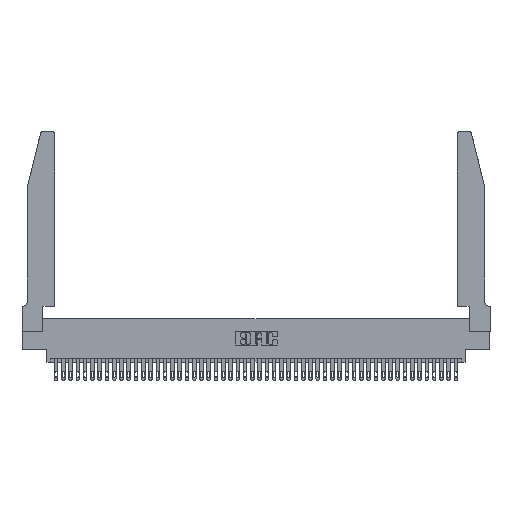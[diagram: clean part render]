
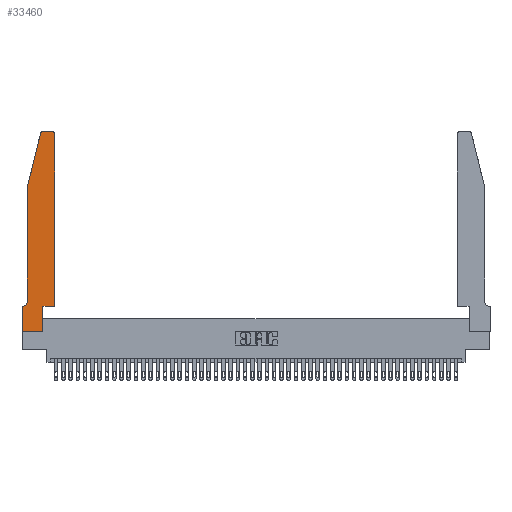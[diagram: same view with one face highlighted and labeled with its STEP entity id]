
A CAD part, top view. The second image highlights one B-rep face of the part: STEP entity #33460.
In plain terms, the highlighted planar face has unit normal (0, 0, 1).
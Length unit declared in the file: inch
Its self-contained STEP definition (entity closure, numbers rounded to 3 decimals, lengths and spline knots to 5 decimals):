
#49 = LINE ( 'NONE', #32958, #11960 ) ;
#180 = DIRECTION ( 'NONE',  ( 0., 0., -1. ) ) ;
#320 = ORIENTED_EDGE ( 'NONE', *, *, #35394, .T. ) ;
#597 = ORIENTED_EDGE ( 'NONE', *, *, #32413, .T. ) ;
#775 = CIRCLE ( 'NONE', #8911, 0.03 ) ;
#868 = CARTESIAN_POINT ( 'NONE',  ( 0.0055, 0.35, 0.37 ) ) ;
#1053 = LINE ( 'NONE', #13685, #38509 ) ;
#1512 = ORIENTED_EDGE ( 'NONE', *, *, #27033, .T. ) ;
#1683 = VERTEX_POINT ( 'NONE', #43651 ) ;
#1830 = CARTESIAN_POINT ( 'NONE',  ( 0., 0., 0.37 ) ) ;
#1929 = CARTESIAN_POINT ( 'NONE',  ( 0.284, 2.72, 0.37 ) ) ;
#2062 = CARTESIAN_POINT ( 'NONE',  ( 0.4505, 2.72, 0.37 ) ) ;
#2100 = DIRECTION ( 'NONE',  ( 0., 0., 1. ) ) ;
#3580 = ORIENTED_EDGE ( 'NONE', *, *, #25906, .T. ) ;
#3643 = VERTEX_POINT ( 'NONE', #4971 ) ;
#4400 = DIRECTION ( 'NONE',  ( 1., 0., 0. ) ) ;
#4857 = LINE ( 'NONE', #1830, #40006 ) ;
#4971 = CARTESIAN_POINT ( 'NONE',  ( 0.25487, 2.72718, 0.37 ) ) ;
#5727 = VERTEX_POINT ( 'NONE', #44080 ) ;
#5959 = EDGE_CURVE ( 'NONE', #5727, #34735, #10338, .T. ) ;
#7249 = VECTOR ( 'NONE', #20449, 39.37008 ) ;
#7508 = CARTESIAN_POINT ( 'NONE',  ( 0.0755, 2., 0.37 ) ) ;
#7820 = EDGE_CURVE ( 'NONE', #31513, #5727, #1053, .T. ) ;
#8633 = DIRECTION ( 'NONE',  ( 0., -1., 0. ) ) ;
#8911 = AXIS2_PLACEMENT_3D ( 'NONE', #1929, #2100, #9671 ) ;
#9350 = VERTEX_POINT ( 'NONE', #10388 ) ;
#9605 = ORIENTED_EDGE ( 'NONE', *, *, #38055, .T. ) ;
#9671 = DIRECTION ( 'NONE',  ( 1., 0., 0. ) ) ;
#10338 = LINE ( 'NONE', #34798, #28529 ) ;
#10388 = CARTESIAN_POINT ( 'NONE',  ( 0., 0.35, 0.37 ) ) ;
#10702 = CARTESIAN_POINT ( 'NONE',  ( 0.0755, 2., 0.37 ) ) ;
#10825 = CIRCLE ( 'NONE', #13218, 0.07 ) ;
#10828 = VECTOR ( 'NONE', #38750, 39.37008 ) ;
#11960 = VECTOR ( 'NONE', #28860, 39.37008 ) ;
#12140 = LINE ( 'NONE', #10702, #19532 ) ;
#12733 = CARTESIAN_POINT ( 'NONE',  ( 0.2865, 0.35, 0.37 ) ) ;
#13218 = AXIS2_PLACEMENT_3D ( 'NONE', #35932, #180, #17667 ) ;
#13668 = LINE ( 'NONE', #16581, #10828 ) ;
#13685 = CARTESIAN_POINT ( 'NONE',  ( 0., 0., 0.37 ) ) ;
#16581 = CARTESIAN_POINT ( 'NONE',  ( 0.2605, 2.75, 0.37 ) ) ;
#17201 = VERTEX_POINT ( 'NONE', #38760 ) ;
#17405 = CARTESIAN_POINT ( 'NONE',  ( 0.4505, 0.35, 0.37 ) ) ;
#17667 = DIRECTION ( 'NONE',  ( -1., 0., 0. ) ) ;
#18306 = LINE ( 'NONE', #42037, #43747 ) ;
#18326 = CARTESIAN_POINT ( 'NONE',  ( 0., 0.35, 0.37 ) ) ;
#19209 = EDGE_CURVE ( 'NONE', #3643, #19293, #12140, .T. ) ;
#19293 = VERTEX_POINT ( 'NONE', #7508 ) ;
#19532 = VECTOR ( 'NONE', #32159, 39.37008 ) ;
#19920 = ORIENTED_EDGE ( 'NONE', *, *, #46606, .T. ) ;
#20341 = ORIENTED_EDGE ( 'NONE', *, *, #26745, .T. ) ;
#20449 = DIRECTION ( 'NONE',  ( 1., 0., 0. ) ) ;
#20710 = CARTESIAN_POINT ( 'NONE',  ( 0.4505, 0.35, 0.37 ) ) ;
#21382 = VERTEX_POINT ( 'NONE', #30533 ) ;
#22530 = ORIENTED_EDGE ( 'NONE', *, *, #7820, .T. ) ;
#22850 = DIRECTION ( 'NONE',  ( 0., 0., 1. ) ) ;
#23179 = CARTESIAN_POINT ( 'NONE',  ( 0.4505, 0.35, 0.37 ) ) ;
#23482 = ORIENTED_EDGE ( 'NONE', *, *, #24258, .T. ) ;
#23630 = LINE ( 'NONE', #20710, #46240 ) ;
#24258 = EDGE_CURVE ( 'NONE', #9350, #31513, #4857, .T. ) ;
#24335 = EDGE_CURVE ( 'NONE', #35291, #46586, #23630, .T. ) ;
#25906 = EDGE_CURVE ( 'NONE', #42373, #9350, #18306, .T. ) ;
#26607 = LINE ( 'NONE', #17405, #7249 ) ;
#26745 = EDGE_CURVE ( 'NONE', #19293, #17201, #49, .T. ) ;
#27018 = CARTESIAN_POINT ( 'NONE',  ( 0.4205, 2.72, 0.37 ) ) ;
#27033 = EDGE_CURVE ( 'NONE', #21382, #1683, #13668, .T. ) ;
#27490 = ORIENTED_EDGE ( 'NONE', *, *, #24335, .T. ) ;
#27534 = EDGE_LOOP ( 'NONE', ( #1512, #320, #35871, #20341, #9605, #3580, #23482, #22530, #41490, #19920, #27490, #597 ) ) ;
#27574 = DIRECTION ( 'NONE',  ( 0., 1., 0. ) ) ;
#28515 = CARTESIAN_POINT ( 'NONE',  ( 0., 0., 0.37 ) ) ;
#28529 = VECTOR ( 'NONE', #27574, 39.37008 ) ;
#28835 = DIRECTION ( 'NONE',  ( 1., 0., 0. ) ) ;
#28860 = DIRECTION ( 'NONE',  ( 0., -1., 0. ) ) ;
#30533 = CARTESIAN_POINT ( 'NONE',  ( 0.4205, 2.75, 0.37 ) ) ;
#31513 = VERTEX_POINT ( 'NONE', #28515 ) ;
#31672 = DIRECTION ( 'NONE',  ( 0., 1., 0. ) ) ;
#32159 = DIRECTION ( 'NONE',  ( -0.239, -0.971, 0. ) ) ;
#32413 = EDGE_CURVE ( 'NONE', #46586, #21382, #35685, .T. ) ;
#32476 = DIRECTION ( 'NONE',  ( 0., 0., 1. ) ) ;
#32958 = CARTESIAN_POINT ( 'NONE',  ( 0.0755, 2., 0.37 ) ) ;
#33460 = ADVANCED_FACE ( 'NONE', ( #46296 ), #36362, .T. ) ;
#34735 = VERTEX_POINT ( 'NONE', #12733 ) ;
#34798 = CARTESIAN_POINT ( 'NONE',  ( 0.2865, 0.35, 0.37 ) ) ;
#35291 = VERTEX_POINT ( 'NONE', #23179 ) ;
#35394 = EDGE_CURVE ( 'NONE', #1683, #3643, #775, .T. ) ;
#35685 = CIRCLE ( 'NONE', #42226, 0.03 ) ;
#35871 = ORIENTED_EDGE ( 'NONE', *, *, #19209, .T. ) ;
#35932 = CARTESIAN_POINT ( 'NONE',  ( 0.0055, 0.42, 0.37 ) ) ;
#36362 = PLANE ( 'NONE',  #45246 ) ;
#38055 = EDGE_CURVE ( 'NONE', #17201, #42373, #10825, .T. ) ;
#38509 = VECTOR ( 'NONE', #4400, 39.37008 ) ;
#38750 = DIRECTION ( 'NONE',  ( -1., 0., 0. ) ) ;
#38760 = CARTESIAN_POINT ( 'NONE',  ( 0.0755, 0.42, 0.37 ) ) ;
#40006 = VECTOR ( 'NONE', #8633, 39.37008 ) ;
#41026 = DIRECTION ( 'NONE',  ( 1., 0., 0. ) ) ;
#41490 = ORIENTED_EDGE ( 'NONE', *, *, #5959, .T. ) ;
#42037 = CARTESIAN_POINT ( 'NONE',  ( 0.0755, 0.35, 0.37 ) ) ;
#42226 = AXIS2_PLACEMENT_3D ( 'NONE', #27018, #22850, #41026 ) ;
#42373 = VERTEX_POINT ( 'NONE', #868 ) ;
#43651 = CARTESIAN_POINT ( 'NONE',  ( 0.284, 2.75, 0.37 ) ) ;
#43747 = VECTOR ( 'NONE', #45643, 39.37008 ) ;
#44080 = CARTESIAN_POINT ( 'NONE',  ( 0.2865, 0., 0.37 ) ) ;
#45246 = AXIS2_PLACEMENT_3D ( 'NONE', #18326, #32476, #28835 ) ;
#45643 = DIRECTION ( 'NONE',  ( -1., 0., 0. ) ) ;
#46240 = VECTOR ( 'NONE', #31672, 39.37008 ) ;
#46296 = FACE_OUTER_BOUND ( 'NONE', #27534, .T. ) ;
#46586 = VERTEX_POINT ( 'NONE', #2062 ) ;
#46606 = EDGE_CURVE ( 'NONE', #34735, #35291, #26607, .T. ) ;
